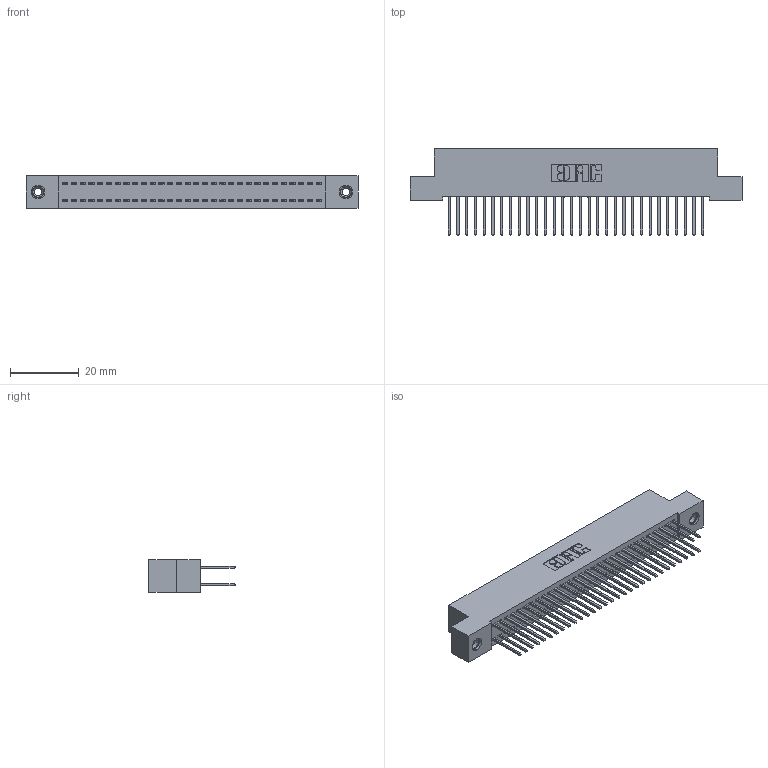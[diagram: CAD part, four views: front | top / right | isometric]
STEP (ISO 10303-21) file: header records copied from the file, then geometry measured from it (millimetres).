
FILE_DESCRIPTION (( 'STEP AP203' ), '1' );
FILE_NAME ('342-060-523-208.STEP', '2019-10-03T13:19:26', ( '' ), ( '' ), 'SwSTEP 2.0', 'SolidWorks 2016', '' );
FILE_SCHEMA (( 'CONFIG_CONTROL_DESIGN' ));
Length unit declared in the file: inch
Products named in the file (4): 345-250-001_345-250-003-102; 345-292-001_345-293-123; 342-060-523-208; 342 Part_TI
Assembly tree (63 placements, depth 2):
  342-060-523-208
    342 Part_TI
    345-292-001_345-293-123  x60
    345-250-001_345-250-003-102  x2
Bounding box: 96.52 x 25.15 x 9.4 mm (x, y, z)
Volume: 8732.8 mm3; surface area: 14452.6 mm2
Topology: 63 solids, 63 shells, 3290 faces, 9735 edges, 6402 vertices
Faces by surface type: plane 2258, cylinder 1016, cone 12, torus 4
Entity records: 21924 total; most frequent: CARTESIAN_POINT 3629, ORIENTED_EDGE 3558, DIRECTION 3153, EDGE_CURVE 1779, VECTOR 1631, LINE 1631, VERTEX_POINT 1180, AXIS2_PLACEMENT_3D 761
